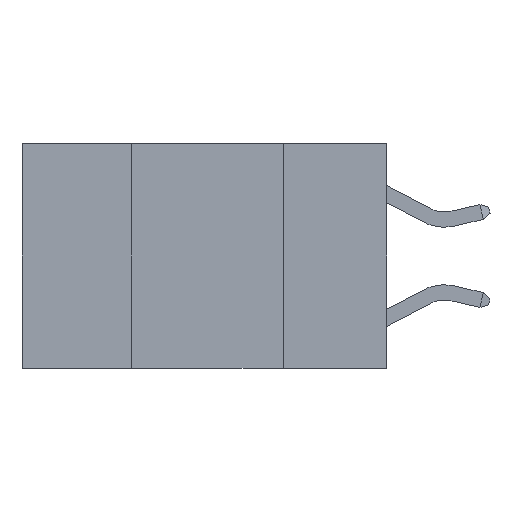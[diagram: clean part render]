
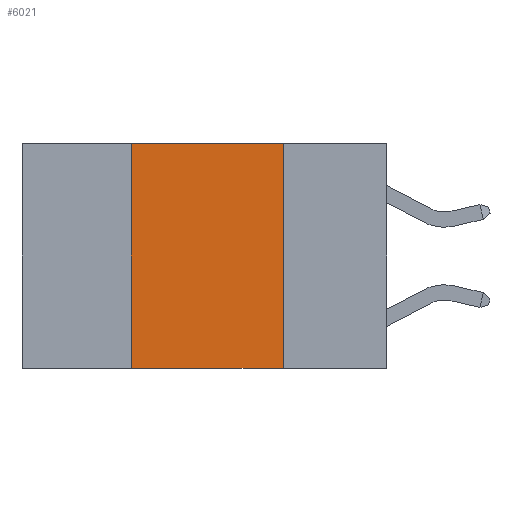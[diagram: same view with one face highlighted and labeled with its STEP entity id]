
A CAD part, left-side view. The second image highlights one B-rep face of the part: STEP entity #6021.
In plain terms, the highlighted planar face has unit normal (-1, 0, 0).
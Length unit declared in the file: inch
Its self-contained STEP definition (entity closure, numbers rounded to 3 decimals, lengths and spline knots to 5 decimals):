
#760 = VECTOR ( 'NONE', #10330, 39.37008 ) ;
#902 = EDGE_CURVE ( 'NONE', #13991, #16050, #17990, .T. ) ;
#1826 = EDGE_CURVE ( 'NONE', #16050, #12648, #15208, .T. ) ;
#1828 = EDGE_CURVE ( 'NONE', #11601, #13991, #15771, .T. ) ;
#1830 = EDGE_CURVE ( 'NONE', #11601, #12648, #10431, .T. ) ;
#1841 = EDGE_LOOP ( 'NONE', ( #19137, #5955, #20209, #20759 ) ) ;
#1923 = VECTOR ( 'NONE', #8516, 39.37008 ) ;
#2508 = CARTESIAN_POINT ( 'NONE',  ( 0., 0.42, -0.37 ) ) ;
#3713 = CARTESIAN_POINT ( 'NONE',  ( 0., 0.42, 0. ) ) ;
#3806 = DIRECTION ( 'NONE',  ( 0., 0., -1. ) ) ;
#4893 = CARTESIAN_POINT ( 'NONE',  ( 0., 0.6, -0.37 ) ) ;
#5955 = ORIENTED_EDGE ( 'NONE', *, *, #902, .F. ) ;
#6021 = ADVANCED_FACE ( 'NONE', ( #13571 ), #7353, .F. ) ;
#7353 = PLANE ( 'NONE',  #8252 ) ;
#8252 = AXIS2_PLACEMENT_3D ( 'NONE', #12806, #14621, #3806 ) ;
#8516 = DIRECTION ( 'NONE',  ( 0., 0., -1. ) ) ;
#10252 = CARTESIAN_POINT ( 'NONE',  ( 0., 0.42, 0. ) ) ;
#10330 = DIRECTION ( 'NONE',  ( 0., 0., 1. ) ) ;
#10431 = LINE ( 'NONE', #4893, #14649 ) ;
#11100 = DIRECTION ( 'NONE',  ( 0., -1., 0. ) ) ;
#11601 = VERTEX_POINT ( 'NONE', #2508 ) ;
#12648 = VERTEX_POINT ( 'NONE', #17826 ) ;
#12681 = VECTOR ( 'NONE', #11100, 39.37008 ) ;
#12806 = CARTESIAN_POINT ( 'NONE',  ( 0., 0.6, 0. ) ) ;
#13571 = FACE_OUTER_BOUND ( 'NONE', #1841, .T. ) ;
#13991 = VERTEX_POINT ( 'NONE', #3713 ) ;
#14621 = DIRECTION ( 'NONE',  ( 1., 0., 0. ) ) ;
#14649 = VECTOR ( 'NONE', #22660, 39.37008 ) ;
#15208 = LINE ( 'NONE', #19205, #1923 ) ;
#15771 = LINE ( 'NONE', #10252, #760 ) ;
#16050 = VERTEX_POINT ( 'NONE', #16949 ) ;
#16949 = CARTESIAN_POINT ( 'NONE',  ( 0., 0.17, 0. ) ) ;
#17826 = CARTESIAN_POINT ( 'NONE',  ( 0., 0.17, -0.37 ) ) ;
#17990 = LINE ( 'NONE', #19995, #12681 ) ;
#19137 = ORIENTED_EDGE ( 'NONE', *, *, #1826, .F. ) ;
#19205 = CARTESIAN_POINT ( 'NONE',  ( 0., 0.17, 0. ) ) ;
#19995 = CARTESIAN_POINT ( 'NONE',  ( 0., 0.6, 0. ) ) ;
#20209 = ORIENTED_EDGE ( 'NONE', *, *, #1828, .F. ) ;
#20759 = ORIENTED_EDGE ( 'NONE', *, *, #1830, .T. ) ;
#22660 = DIRECTION ( 'NONE',  ( 0., -1., 0. ) ) ;
